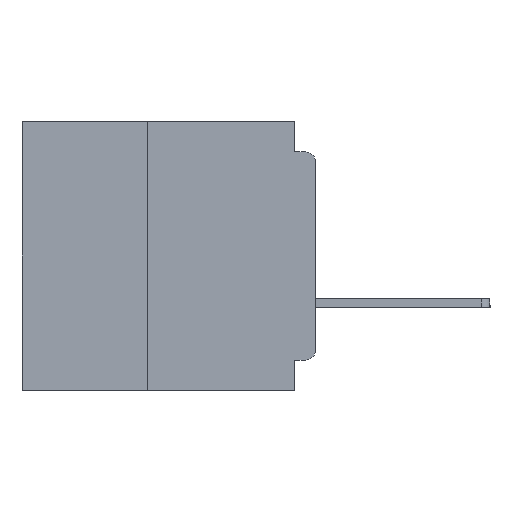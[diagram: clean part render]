
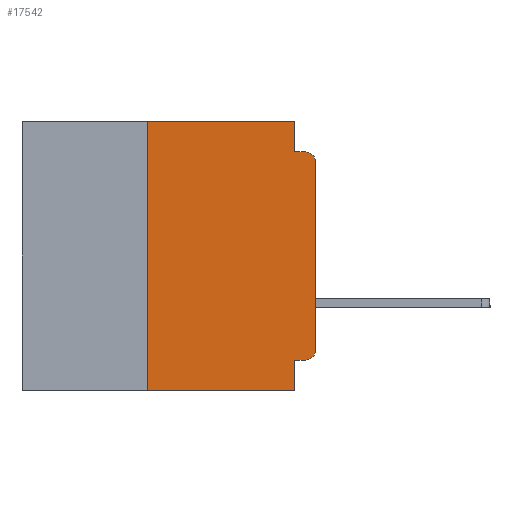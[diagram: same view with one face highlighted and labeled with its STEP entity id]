
A CAD part, left-side view. The second image highlights one B-rep face of the part: STEP entity #17542.
In plain terms, the highlighted planar face has unit normal (-1, 0, 0).
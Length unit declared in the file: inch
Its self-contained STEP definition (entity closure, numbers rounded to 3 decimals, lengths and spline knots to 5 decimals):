
#259 = DIRECTION ( 'NONE',  ( 0., 0., -1. ) ) ;
#836 = ORIENTED_EDGE ( 'NONE', *, *, #1538, .T. ) ;
#846 = LINE ( 'NONE', #29219, #31292 ) ;
#1305 = VERTEX_POINT ( 'NONE', #19333 ) ;
#1538 = EDGE_CURVE ( 'NONE', #17236, #1305, #35507, .T. ) ;
#1857 = CARTESIAN_POINT ( 'NONE',  ( 0., 0.031, -0.4 ) ) ;
#2271 = EDGE_CURVE ( 'NONE', #23721, #10610, #24428, .T. ) ;
#2463 = CARTESIAN_POINT ( 'NONE',  ( 0., 0.25, -0.4 ) ) ;
#2558 = CARTESIAN_POINT ( 'NONE',  ( 0., 0.437, -0.4 ) ) ;
#2709 = VECTOR ( 'NONE', #32075, 39.37008 ) ;
#2863 = DIRECTION ( 'NONE',  ( 0., 0., -1. ) ) ;
#2922 = ORIENTED_EDGE ( 'NONE', *, *, #2271, .F. ) ;
#5802 = VECTOR ( 'NONE', #28404, 39.37008 ) ;
#6095 = LINE ( 'NONE', #8485, #28735 ) ;
#6388 = ORIENTED_EDGE ( 'NONE', *, *, #21028, .T. ) ;
#7441 = CIRCLE ( 'NONE', #32888, 0.015 ) ;
#7475 = VECTOR ( 'NONE', #10654, 39.37008 ) ;
#7504 = CARTESIAN_POINT ( 'NONE',  ( 0., 0., 0. ) ) ;
#7698 = CARTESIAN_POINT ( 'NONE',  ( 0., 0.437, 0. ) ) ;
#7791 = VERTEX_POINT ( 'NONE', #34376 ) ;
#8331 = ORIENTED_EDGE ( 'NONE', *, *, #26328, .F. ) ;
#8485 = CARTESIAN_POINT ( 'NONE',  ( 0., 0.031, 0. ) ) ;
#10610 = VERTEX_POINT ( 'NONE', #36393 ) ;
#10654 = DIRECTION ( 'NONE',  ( 0., -1., 0. ) ) ;
#10947 = VERTEX_POINT ( 'NONE', #37915 ) ;
#11420 = LINE ( 'NONE', #2558, #2709 ) ;
#11438 = DIRECTION ( 'NONE',  ( 0., 0., -1. ) ) ;
#12078 = EDGE_CURVE ( 'NONE', #10947, #16846, #16265, .T. ) ;
#12543 = EDGE_CURVE ( 'NONE', #23721, #30653, #7441, .T. ) ;
#13025 = EDGE_CURVE ( 'NONE', #7791, #10947, #35990, .T. ) ;
#13375 = AXIS2_PLACEMENT_3D ( 'NONE', #22382, #20322, #20181 ) ;
#14266 = DIRECTION ( 'NONE',  ( 0., 0., 1. ) ) ;
#16265 = LINE ( 'NONE', #7698, #7475 ) ;
#16548 = VECTOR ( 'NONE', #31979, 39.37008 ) ;
#16846 = VERTEX_POINT ( 'NONE', #32361 ) ;
#17054 = EDGE_LOOP ( 'NONE', ( #24945, #836, #25699, #37182, #19642, #28707, #6388, #8331, #2922, #26775 ) ) ;
#17236 = VERTEX_POINT ( 'NONE', #19434 ) ;
#17445 = DIRECTION ( 'NONE',  ( 0., -1., 0. ) ) ;
#17542 = ADVANCED_FACE ( 'NONE', ( #28818 ), #32561, .F. ) ;
#17863 = DIRECTION ( 'NONE',  ( 1., 0., 0. ) ) ;
#19333 = CARTESIAN_POINT ( 'NONE',  ( 0., 0.015, -0.045 ) ) ;
#19434 = CARTESIAN_POINT ( 'NONE',  ( 0., 0., -0.06 ) ) ;
#19642 = ORIENTED_EDGE ( 'NONE', *, *, #12078, .F. ) ;
#20181 = DIRECTION ( 'NONE',  ( 0., 0., -1. ) ) ;
#20322 = DIRECTION ( 'NONE',  ( -1., 0., 0. ) ) ;
#20343 = VECTOR ( 'NONE', #14266, 39.37008 ) ;
#20505 = DIRECTION ( 'NONE',  ( -1., 0., 0. ) ) ;
#21028 = EDGE_CURVE ( 'NONE', #7791, #22130, #11420, .T. ) ;
#22130 = VERTEX_POINT ( 'NONE', #31483 ) ;
#22382 = CARTESIAN_POINT ( 'NONE',  ( 0., 0.015, -0.06 ) ) ;
#23634 = LINE ( 'NONE', #7504, #30530 ) ;
#23721 = VERTEX_POINT ( 'NONE', #27652 ) ;
#24241 = VERTEX_POINT ( 'NONE', #27029 ) ;
#24428 = LINE ( 'NONE', #32015, #16548 ) ;
#24945 = ORIENTED_EDGE ( 'NONE', *, *, #34744, .T. ) ;
#25699 = ORIENTED_EDGE ( 'NONE', *, *, #30812, .F. ) ;
#26328 = EDGE_CURVE ( 'NONE', #10610, #22130, #37131, .T. ) ;
#26775 = ORIENTED_EDGE ( 'NONE', *, *, #12543, .T. ) ;
#27029 = CARTESIAN_POINT ( 'NONE',  ( 0., 0.031, -0.045 ) ) ;
#27652 = CARTESIAN_POINT ( 'NONE',  ( 0., 0.015, -0.355 ) ) ;
#28404 = DIRECTION ( 'NONE',  ( 0., 0., -1. ) ) ;
#28707 = ORIENTED_EDGE ( 'NONE', *, *, #13025, .F. ) ;
#28735 = VECTOR ( 'NONE', #11438, 39.37008 ) ;
#28818 = FACE_OUTER_BOUND ( 'NONE', #17054, .T. ) ;
#29219 = CARTESIAN_POINT ( 'NONE',  ( 0., 0., -0.045 ) ) ;
#30530 = VECTOR ( 'NONE', #31141, 39.37008 ) ;
#30653 = VERTEX_POINT ( 'NONE', #34321 ) ;
#30812 = EDGE_CURVE ( 'NONE', #24241, #1305, #846, .T. ) ;
#31141 = DIRECTION ( 'NONE',  ( 0., 0., 1. ) ) ;
#31292 = VECTOR ( 'NONE', #17445, 39.37008 ) ;
#31483 = CARTESIAN_POINT ( 'NONE',  ( 0., 0.031, -0.4 ) ) ;
#31979 = DIRECTION ( 'NONE',  ( 0., 1., 0. ) ) ;
#32015 = CARTESIAN_POINT ( 'NONE',  ( 0., 0., -0.355 ) ) ;
#32075 = DIRECTION ( 'NONE',  ( 0., -1., 0. ) ) ;
#32361 = CARTESIAN_POINT ( 'NONE',  ( 0., 0.031, 0. ) ) ;
#32561 = PLANE ( 'NONE',  #32777 ) ;
#32777 = AXIS2_PLACEMENT_3D ( 'NONE', #35509, #17863, #259 ) ;
#32888 = AXIS2_PLACEMENT_3D ( 'NONE', #38116, #20505, #2863 ) ;
#33662 = EDGE_CURVE ( 'NONE', #16846, #24241, #6095, .T. ) ;
#34321 = CARTESIAN_POINT ( 'NONE',  ( 0., 0., -0.34 ) ) ;
#34376 = CARTESIAN_POINT ( 'NONE',  ( 0., 0.25, -0.4 ) ) ;
#34744 = EDGE_CURVE ( 'NONE', #30653, #17236, #23634, .T. ) ;
#35507 = CIRCLE ( 'NONE', #13375, 0.015 ) ;
#35509 = CARTESIAN_POINT ( 'NONE',  ( 0., 0.437, 0. ) ) ;
#35990 = LINE ( 'NONE', #2463, #20343 ) ;
#36393 = CARTESIAN_POINT ( 'NONE',  ( 0., 0.031, -0.355 ) ) ;
#37131 = LINE ( 'NONE', #1857, #5802 ) ;
#37182 = ORIENTED_EDGE ( 'NONE', *, *, #33662, .F. ) ;
#37915 = CARTESIAN_POINT ( 'NONE',  ( 0., 0.25, 0. ) ) ;
#38116 = CARTESIAN_POINT ( 'NONE',  ( 0., 0.015, -0.34 ) ) ;
